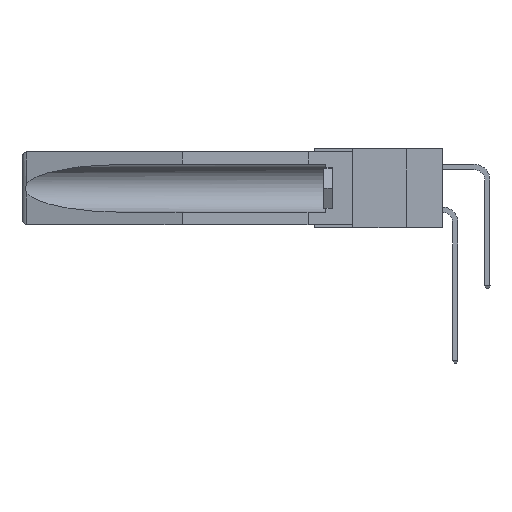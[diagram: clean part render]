
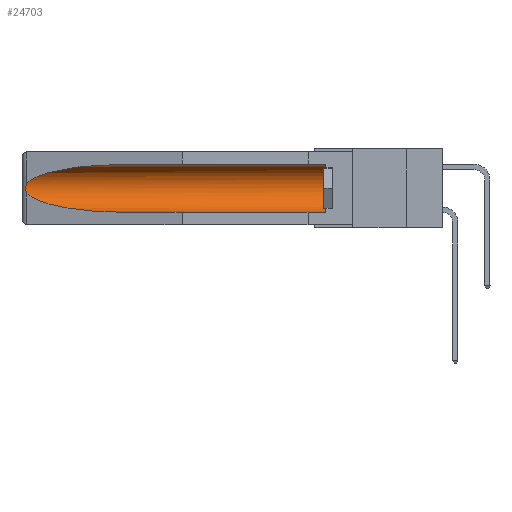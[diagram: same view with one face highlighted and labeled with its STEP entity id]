
A CAD part, left-side view. The second image highlights one B-rep face of the part: STEP entity #24703.
In plain terms, the highlighted cylindrical face has radius 2.857 mm (diameter 5.715 mm), a partial arc.
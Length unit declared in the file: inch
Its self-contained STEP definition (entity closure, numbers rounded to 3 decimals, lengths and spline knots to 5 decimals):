
#55 = ORIENTED_EDGE ( 'NONE', *, *, #4184, .T. ) ;
#63 = FACE_OUTER_BOUND ( 'NONE', #22888, .T. ) ;
#139 = EDGE_CURVE ( 'NONE', #6269, #11017, #17182, .T. ) ;
#499 = CARTESIAN_POINT ( 'NONE',  ( 0.26537, 1.52718, -0.14972 ) ) ;
#555 = ORIENTED_EDGE ( 'NONE', *, *, #22973, .T. ) ;
#2357 = VERTEX_POINT ( 'NONE', #18153 ) ;
#2521 = CYLINDRICAL_SURFACE ( 'NONE', #13619, 0.1125 ) ;
#2583 = CARTESIAN_POINT ( 'NONE',  ( 0.26537, 1.52718, -0.19328 ) ) ;
#3562 = EDGE_CURVE ( 'NONE', #9892, #2357, #10831, .T. ) ;
#4142 = CARTESIAN_POINT ( 'NONE',  ( 0.155, -0.30754, -0.059 ) ) ;
#4184 = EDGE_CURVE ( 'NONE', #2357, #5218, #17509, .T. ) ;
#4964 = DIRECTION ( 'NONE',  ( 0., 1., 0. ) ) ;
#4991 = CARTESIAN_POINT ( 'NONE',  ( 0.26537, 1.52718, -0.14972 ) ) ;
#5218 = VERTEX_POINT ( 'NONE', #4991 ) ;
#5475 = CARTESIAN_POINT ( 'NONE',  ( 0.155, 0.126, -0.284 ) ) ;
#5546 = ORIENTED_EDGE ( 'NONE', *, *, #3562, .T. ) ;
#5662 = EDGE_CURVE ( 'NONE', #8599, #11017, #10282, .T. ) ;
#5983 = CARTESIAN_POINT ( 'NONE',  ( 0.25451, 1.48313, -0.24835 ) ) ;
#6269 = VERTEX_POINT ( 'NONE', #24032 ) ;
#6525 = CARTESIAN_POINT ( 'NONE',  ( 0.2673, 1.5327, -0.16383 ) ) ;
#6703 = CARTESIAN_POINT ( 'NONE',  ( 0.155, -0.30754, -0.284 ) ) ;
#6791 = CARTESIAN_POINT ( 'NONE',  ( 0.26537, 1.52718, -0.14972 ) ) ;
#7839 = EDGE_CURVE ( 'NONE', #8599, #9892, #19087, .T. ) ;
#7999 = CARTESIAN_POINT ( 'NONE',  ( 0.21114, 1.30732, -0.284 ) ) ;
#8599 = VERTEX_POINT ( 'NONE', #5475 ) ;
#8889 = ORIENTED_EDGE ( 'NONE', *, *, #139, .T. ) ;
#9892 = VERTEX_POINT ( 'NONE', #11097 ) ;
#10196 = CARTESIAN_POINT ( 'NONE',  ( 0.21114, 1.30732, -0.059 ) ) ;
#10282 = LINE ( 'NONE', #6703, #18909 ) ;
#10740 = CARTESIAN_POINT ( 'NONE',  ( 0.2675, 1.53308, -0.16763 ) ) ;
#10831 = LINE ( 'NONE', #4142, #14546 ) ;
#11017 = VERTEX_POINT ( 'NONE', #14515 ) ;
#11097 = CARTESIAN_POINT ( 'NONE',  ( 0.155, 0.126, -0.059 ) ) ;
#11686 = CARTESIAN_POINT ( 'NONE',  ( 0.155, -0.30754, -0.1715 ) ) ;
#12715 = CARTESIAN_POINT ( 'NONE',  ( 0.26597, 1.5296, -0.19026 ) ) ;
#13173 = DIRECTION ( 'NONE',  ( 0., 0., 1. ) ) ;
#13265 = DIRECTION ( 'NONE',  ( 0., -1., 0. ) ) ;
#13619 = AXIS2_PLACEMENT_3D ( 'NONE', #11686, #25326, #17639 ) ;
#13946 = DIRECTION ( 'NONE',  ( 0., 1., 0. ) ) ;
#14515 = CARTESIAN_POINT ( 'NONE',  ( 0.155, 1.07973, -0.284 ) ) ;
#14546 = VECTOR ( 'NONE', #13946, 39.37008 ) ;
#15982 = CARTESIAN_POINT ( 'NONE',  ( 0.25451, 1.48313, -0.09465 ) ) ;
#16506 = ORIENTED_EDGE ( 'NONE', *, *, #7839, .T. ) ;
#16966 = CARTESIAN_POINT ( 'NONE',  ( 0.155, 0.126, -0.1715 ) ) ;
#17182 =( BOUNDED_CURVE ( )  B_SPLINE_CURVE ( 3, ( #21612, #5983, #7999, #21698 ),
 .UNSPECIFIED., .F., .F. ) 
 B_SPLINE_CURVE_WITH_KNOTS ( ( 4, 4 ),
 ( 0.1948, 1.5708 ),
 .UNSPECIFIED. ) 
 CURVE ( )  GEOMETRIC_REPRESENTATION_ITEM ( )  RATIONAL_B_SPLINE_CURVE ( ( 1., 0.848, 0.848, 1. ) ) 
 REPRESENTATION_ITEM ( '' )  );
#17509 =( BOUNDED_CURVE ( )  B_SPLINE_CURVE ( 3, ( #18131, #10196, #15982, #499 ),
 .UNSPECIFIED., .F., .F. ) 
 B_SPLINE_CURVE_WITH_KNOTS ( ( 4, 4 ),
 ( 4.71239, 6.08839 ),
 .UNSPECIFIED. ) 
 CURVE ( )  GEOMETRIC_REPRESENTATION_ITEM ( )  RATIONAL_B_SPLINE_CURVE ( ( 1., 0.848, 0.848, 1. ) ) 
 REPRESENTATION_ITEM ( '' )  );
#17639 = DIRECTION ( 'NONE',  ( 0., 0., 1. ) ) ;
#18131 = CARTESIAN_POINT ( 'NONE',  ( 0.155, 1.07973, -0.059 ) ) ;
#18153 = CARTESIAN_POINT ( 'NONE',  ( 0.155, 1.07973, -0.059 ) ) ;
#18909 = VECTOR ( 'NONE', #4964, 39.37008 ) ;
#19087 = CIRCLE ( 'NONE', #22715, 0.1125 ) ;
#20184 = CARTESIAN_POINT ( 'NONE',  ( 0.26654, 1.53092, -0.15636 ) ) ;
#21612 = CARTESIAN_POINT ( 'NONE',  ( 0.26537, 1.52718, -0.19328 ) ) ;
#21698 = CARTESIAN_POINT ( 'NONE',  ( 0.155, 1.07973, -0.284 ) ) ;
#22064 = ORIENTED_EDGE ( 'NONE', *, *, #5662, .F. ) ;
#22291 = CARTESIAN_POINT ( 'NONE',  ( 0.2675, 1.53308, -0.17534 ) ) ;
#22444 = CARTESIAN_POINT ( 'NONE',  ( 0.26597, 1.52961, -0.15275 ) ) ;
#22715 = AXIS2_PLACEMENT_3D ( 'NONE', #16966, #13265, #13173 ) ;
#22888 = EDGE_LOOP ( 'NONE', ( #55, #555, #8889, #22064, #16506, #5546 ) ) ;
#22918 = B_SPLINE_CURVE_WITH_KNOTS ( 'NONE', 3,
 ( #6791, #22444, #20184, #6525, #10740, #22291, #24060, #24399, #12715, #2583 ),
 .UNSPECIFIED., .F., .F.,
 ( 4, 2, 2, 2, 4 ),
 ( 0., 0.00029, 0.00058, 0.00087, 0.00117 ),
 .UNSPECIFIED. ) ;
#22973 = EDGE_CURVE ( 'NONE', #5218, #6269, #22918, .T. ) ;
#24032 = CARTESIAN_POINT ( 'NONE',  ( 0.26537, 1.52718, -0.19328 ) ) ;
#24060 = CARTESIAN_POINT ( 'NONE',  ( 0.2673, 1.53269, -0.17917 ) ) ;
#24399 = CARTESIAN_POINT ( 'NONE',  ( 0.26655, 1.53094, -0.18657 ) ) ;
#24703 = ADVANCED_FACE ( 'NONE', ( #63 ), #2521, .F. ) ;
#25326 = DIRECTION ( 'NONE',  ( 0., 1., 0. ) ) ;
